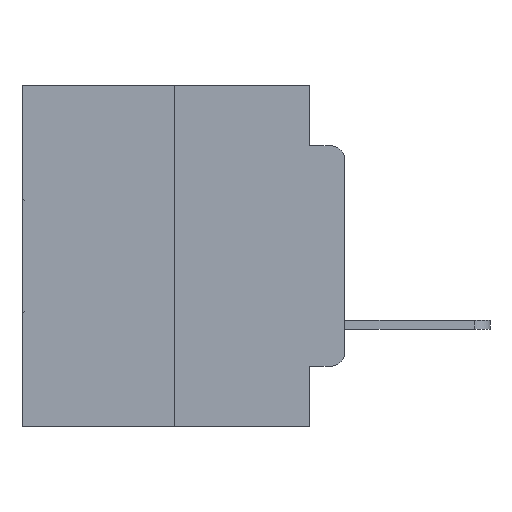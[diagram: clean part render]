
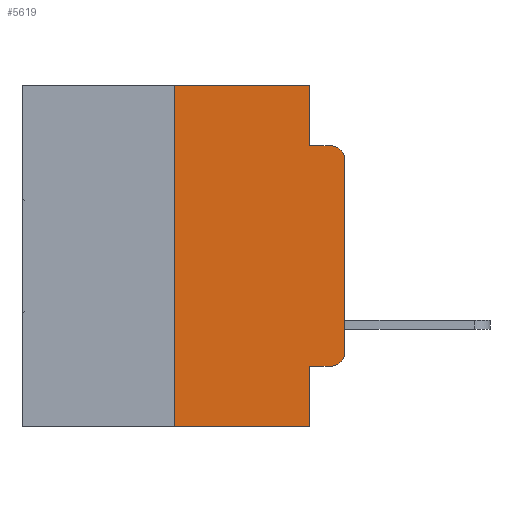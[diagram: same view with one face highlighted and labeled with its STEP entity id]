
A CAD part, left-side view. The second image highlights one B-rep face of the part: STEP entity #5619.
In plain terms, the highlighted planar face has unit normal (-1, 0, 0).
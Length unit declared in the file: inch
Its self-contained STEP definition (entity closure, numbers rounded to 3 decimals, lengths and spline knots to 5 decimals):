
#1913 = LINE ( 'NONE', #23528, #25147 ) ;
#1971 = ORIENTED_EDGE ( 'NONE', *, *, #14419, .T. ) ;
#2169 = CARTESIAN_POINT ( 'NONE',  ( 0., 0.051, 0. ) ) ;
#2728 = ORIENTED_EDGE ( 'NONE', *, *, #17407, .F. ) ;
#2866 = CARTESIAN_POINT ( 'NONE',  ( 0., 0.02, -0.1085 ) ) ;
#3469 = CARTESIAN_POINT ( 'NONE',  ( 0., 0.02, -0.3915 ) ) ;
#4082 = VECTOR ( 'NONE', #23104, 39.37008 ) ;
#4617 = CARTESIAN_POINT ( 'NONE',  ( 0., 0.473, 0. ) ) ;
#4998 = VERTEX_POINT ( 'NONE', #2169 ) ;
#5328 = AXIS2_PLACEMENT_3D ( 'NONE', #2866, #7622, #26250 ) ;
#5439 = DIRECTION ( 'NONE',  ( 0., -1., 0. ) ) ;
#5619 = ADVANCED_FACE ( 'NONE', ( #25161 ), #28362, .F. ) ;
#6384 = VECTOR ( 'NONE', #13689, 39.37008 ) ;
#7258 = CIRCLE ( 'NONE', #5328, 0.02 ) ;
#7494 = VECTOR ( 'NONE', #5439, 39.37008 ) ;
#7622 = DIRECTION ( 'NONE',  ( -1., 0., 0. ) ) ;
#8025 = VECTOR ( 'NONE', #26935, 39.37008 ) ;
#8182 = VERTEX_POINT ( 'NONE', #19626 ) ;
#8213 = VECTOR ( 'NONE', #14783, 39.37008 ) ;
#8399 = LINE ( 'NONE', #26500, #23142 ) ;
#8420 = DIRECTION ( 'NONE',  ( -1., 0., 0. ) ) ;
#8676 = CARTESIAN_POINT ( 'NONE',  ( 0., 0., -0.3915 ) ) ;
#8894 = CARTESIAN_POINT ( 'NONE',  ( 0., 0.473, 0. ) ) ;
#9388 = EDGE_CURVE ( 'NONE', #24673, #11582, #17977, .T. ) ;
#10350 = LINE ( 'NONE', #8894, #4082 ) ;
#10823 = CARTESIAN_POINT ( 'NONE',  ( 0., 0.25, -0.5 ) ) ;
#11365 = VERTEX_POINT ( 'NONE', #26682 ) ;
#11464 = EDGE_LOOP ( 'NONE', ( #1971, #20919, #18676, #22424, #2728, #30117, #12405, #12609, #15873, #30423 ) ) ;
#11582 = VERTEX_POINT ( 'NONE', #8676 ) ;
#11992 = CARTESIAN_POINT ( 'NONE',  ( 0., 0.02, -0.4115 ) ) ;
#12405 = ORIENTED_EDGE ( 'NONE', *, *, #26221, .T. ) ;
#12411 = CARTESIAN_POINT ( 'NONE',  ( 0., 0.051, 0. ) ) ;
#12609 = ORIENTED_EDGE ( 'NONE', *, *, #18958, .F. ) ;
#12794 = VERTEX_POINT ( 'NONE', #26997 ) ;
#12972 = VERTEX_POINT ( 'NONE', #10823 ) ;
#13395 = AXIS2_PLACEMENT_3D ( 'NONE', #4617, #21129, #14163 ) ;
#13660 = VERTEX_POINT ( 'NONE', #23854 ) ;
#13689 = DIRECTION ( 'NONE',  ( 0., 0., 1. ) ) ;
#14163 = DIRECTION ( 'NONE',  ( 0., 0., -1. ) ) ;
#14248 = LINE ( 'NONE', #12411, #8025 ) ;
#14411 = LINE ( 'NONE', #26540, #8213 ) ;
#14419 = EDGE_CURVE ( 'NONE', #11582, #8182, #14411, .T. ) ;
#14778 = CARTESIAN_POINT ( 'NONE',  ( 0., 0.473, -0.5 ) ) ;
#14783 = DIRECTION ( 'NONE',  ( 0., 0., 1. ) ) ;
#14821 = LINE ( 'NONE', #15997, #6384 ) ;
#15873 = ORIENTED_EDGE ( 'NONE', *, *, #28491, .T. ) ;
#15997 = CARTESIAN_POINT ( 'NONE',  ( 0., 0.25, 0. ) ) ;
#17191 = CARTESIAN_POINT ( 'NONE',  ( 0., 0.051, -0.5 ) ) ;
#17407 = EDGE_CURVE ( 'NONE', #11365, #4998, #10350, .T. ) ;
#17977 = CIRCLE ( 'NONE', #23574, 0.02 ) ;
#18676 = ORIENTED_EDGE ( 'NONE', *, *, #27300, .F. ) ;
#18895 = VERTEX_POINT ( 'NONE', #17191 ) ;
#18958 = EDGE_CURVE ( 'NONE', #21270, #18895, #14248, .T. ) ;
#19626 = CARTESIAN_POINT ( 'NONE',  ( 0., 0., -0.1085 ) ) ;
#19959 = DIRECTION ( 'NONE',  ( 0., 0., -1. ) ) ;
#20919 = ORIENTED_EDGE ( 'NONE', *, *, #28894, .T. ) ;
#20973 = DIRECTION ( 'NONE',  ( 0., -1., 0. ) ) ;
#21129 = DIRECTION ( 'NONE',  ( 1., 0., 0. ) ) ;
#21270 = VERTEX_POINT ( 'NONE', #24169 ) ;
#22424 = ORIENTED_EDGE ( 'NONE', *, *, #23509, .F. ) ;
#23104 = DIRECTION ( 'NONE',  ( 0., -1., 0. ) ) ;
#23142 = VECTOR ( 'NONE', #24045, 39.37008 ) ;
#23340 = LINE ( 'NONE', #14778, #7494 ) ;
#23509 = EDGE_CURVE ( 'NONE', #4998, #13660, #8399, .T. ) ;
#23528 = CARTESIAN_POINT ( 'NONE',  ( 0., 0.051, -0.0885 ) ) ;
#23574 = AXIS2_PLACEMENT_3D ( 'NONE', #3469, #8420, #19959 ) ;
#23854 = CARTESIAN_POINT ( 'NONE',  ( 0., 0.051, -0.0885 ) ) ;
#24045 = DIRECTION ( 'NONE',  ( 0., 0., -1. ) ) ;
#24169 = CARTESIAN_POINT ( 'NONE',  ( 0., 0.051, -0.4115 ) ) ;
#24673 = VERTEX_POINT ( 'NONE', #11992 ) ;
#25147 = VECTOR ( 'NONE', #20973, 39.37008 ) ;
#25161 = FACE_OUTER_BOUND ( 'NONE', #11464, .T. ) ;
#25961 = EDGE_CURVE ( 'NONE', #12972, #11365, #14821, .T. ) ;
#26221 = EDGE_CURVE ( 'NONE', #12972, #18895, #23340, .T. ) ;
#26250 = DIRECTION ( 'NONE',  ( 0., 0., -1. ) ) ;
#26485 = VECTOR ( 'NONE', #28634, 39.37008 ) ;
#26500 = CARTESIAN_POINT ( 'NONE',  ( 0., 0.051, 0. ) ) ;
#26540 = CARTESIAN_POINT ( 'NONE',  ( 0., 0., 0. ) ) ;
#26682 = CARTESIAN_POINT ( 'NONE',  ( 0., 0.25, 0. ) ) ;
#26935 = DIRECTION ( 'NONE',  ( 0., 0., -1. ) ) ;
#26997 = CARTESIAN_POINT ( 'NONE',  ( 0., 0.02, -0.0885 ) ) ;
#27242 = LINE ( 'NONE', #28734, #26485 ) ;
#27300 = EDGE_CURVE ( 'NONE', #13660, #12794, #1913, .T. ) ;
#28362 = PLANE ( 'NONE',  #13395 ) ;
#28491 = EDGE_CURVE ( 'NONE', #21270, #24673, #27242, .T. ) ;
#28634 = DIRECTION ( 'NONE',  ( 0., -1., 0. ) ) ;
#28734 = CARTESIAN_POINT ( 'NONE',  ( 0., 0.051, -0.4115 ) ) ;
#28894 = EDGE_CURVE ( 'NONE', #8182, #12794, #7258, .T. ) ;
#30117 = ORIENTED_EDGE ( 'NONE', *, *, #25961, .F. ) ;
#30423 = ORIENTED_EDGE ( 'NONE', *, *, #9388, .T. ) ;
